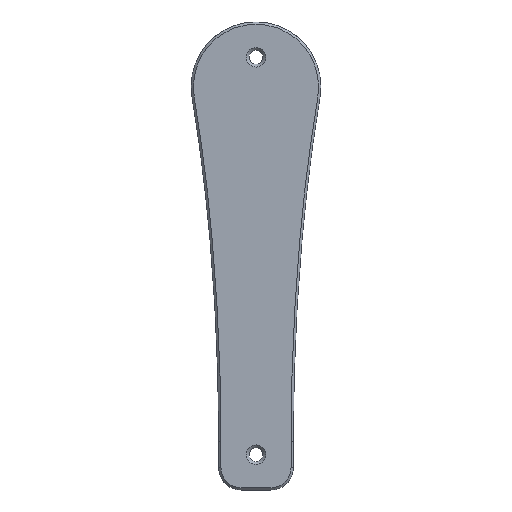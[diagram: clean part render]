
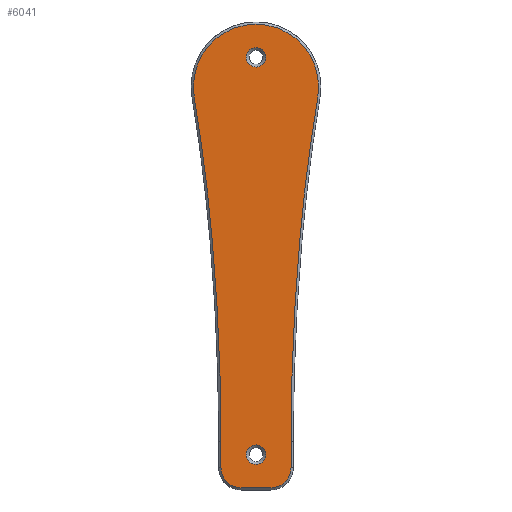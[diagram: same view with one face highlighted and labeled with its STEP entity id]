
A CAD part, front view. The second image highlights one B-rep face of the part: STEP entity #6041.
In plain terms, the highlighted planar face has unit normal (0, -1, 0).
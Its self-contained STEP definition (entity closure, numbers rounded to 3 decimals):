
#19=FACE_BOUND('',#829,.T.);
#20=FACE_BOUND('',#830,.T.);
#27=PLANE('',#6511);
#62=LINE('',#8183,#188);
#66=LINE('',#8195,#192);
#69=LINE('',#8206,#195);
#188=VECTOR('',#6938,10.);
#192=VECTOR('',#6950,10.);
#195=VECTOR('',#6961,10.);
#397=FACE_OUTER_BOUND('',#828,.T.);
#828=EDGE_LOOP('',(#3836,#3837,#3838,#3839,#3840,#3841,#3842,#3843,#3844,
#3845));
#829=EDGE_LOOP('',(#3846));
#830=EDGE_LOOP('',(#3847));
#1817=CIRCLE('',#6482,16.81);
#1820=CIRCLE('',#6486,500.6);
#1821=CIRCLE('',#6488,624.432);
#1824=CIRCLE('',#6493,5.4);
#1825=CIRCLE('',#6496,5.4);
#1828=CIRCLE('',#6501,624.432);
#1829=CIRCLE('',#6503,500.6);
#1832=CIRCLE('',#6512,2.6);
#1833=CIRCLE('',#6513,2.6);
#2138=VERTEX_POINT('',#8159);
#2139=VERTEX_POINT('',#8161);
#2142=VERTEX_POINT('',#8169);
#2144=VERTEX_POINT('',#8174);
#2146=VERTEX_POINT('',#8181);
#2148=VERTEX_POINT('',#8187);
#2150=VERTEX_POINT('',#8193);
#2152=VERTEX_POINT('',#8198);
#2154=VERTEX_POINT('',#8204);
#2156=VERTEX_POINT('',#8211);
#2207=VERTEX_POINT('',#8490);
#2208=VERTEX_POINT('',#8492);
#2718=EDGE_CURVE('',#2138,#2139,#1817,.T.);
#2723=EDGE_CURVE('',#2142,#2138,#1820,.T.);
#2725=EDGE_CURVE('',#2144,#2142,#1821,.T.);
#2729=EDGE_CURVE('',#2146,#2144,#62,.T.);
#2732=EDGE_CURVE('',#2148,#2146,#1824,.T.);
#2735=EDGE_CURVE('',#2150,#2148,#66,.T.);
#2737=EDGE_CURVE('',#2152,#2150,#1825,.T.);
#2740=EDGE_CURVE('',#2154,#2152,#69,.T.);
#2744=EDGE_CURVE('',#2156,#2154,#1828,.T.);
#2745=EDGE_CURVE('',#2139,#2156,#1829,.T.);
#2802=EDGE_CURVE('',#2207,#2207,#1832,.T.);
#2803=EDGE_CURVE('',#2208,#2208,#1833,.T.);
#3836=ORIENTED_EDGE('',*,*,#2718,.F.);
#3837=ORIENTED_EDGE('',*,*,#2723,.F.);
#3838=ORIENTED_EDGE('',*,*,#2725,.F.);
#3839=ORIENTED_EDGE('',*,*,#2729,.F.);
#3840=ORIENTED_EDGE('',*,*,#2732,.F.);
#3841=ORIENTED_EDGE('',*,*,#2735,.F.);
#3842=ORIENTED_EDGE('',*,*,#2737,.F.);
#3843=ORIENTED_EDGE('',*,*,#2740,.F.);
#3844=ORIENTED_EDGE('',*,*,#2744,.F.);
#3845=ORIENTED_EDGE('',*,*,#2745,.F.);
#3846=ORIENTED_EDGE('',*,*,#2802,.F.);
#3847=ORIENTED_EDGE('',*,*,#2803,.F.);
#6041=ADVANCED_FACE('',(#397,#19,#20),#27,.F.);
#6482=AXIS2_PLACEMENT_3D('',#8162,#6915,#6916);
#6486=AXIS2_PLACEMENT_3D('',#8171,#6925,#6926);
#6488=AXIS2_PLACEMENT_3D('',#8176,#6930,#6931);
#6493=AXIS2_PLACEMENT_3D('',#8189,#6944,#6945);
#6496=AXIS2_PLACEMENT_3D('',#8200,#6954,#6955);
#6501=AXIS2_PLACEMENT_3D('',#8213,#6968,#6969);
#6503=AXIS2_PLACEMENT_3D('',#8215,#6972,#6973);
#6511=AXIS2_PLACEMENT_3D('',#8489,#6995,#6996);
#6512=AXIS2_PLACEMENT_3D('',#8491,#6997,#6998);
#6513=AXIS2_PLACEMENT_3D('',#8493,#6999,#7000);
#6915=DIRECTION('center_axis',(0.,1.,0.));
#6916=DIRECTION('ref_axis',(-0.518,0.,0.856));
#6925=DIRECTION('center_axis',(0.,-1.,0.));
#6926=DIRECTION('ref_axis',(0.992,0.,0.125));
#6930=DIRECTION('center_axis',(0.,-1.,0.));
#6931=DIRECTION('ref_axis',(0.99,0.,0.143));
#6938=DIRECTION('',(0.,0.,1.));
#6944=DIRECTION('center_axis',(0.,1.,0.));
#6945=DIRECTION('ref_axis',(-0.707,0.,-0.707));
#6950=DIRECTION('',(-1.,0.,0.));
#6954=DIRECTION('center_axis',(0.,1.,0.));
#6955=DIRECTION('ref_axis',(0.707,0.,-0.707));
#6961=DIRECTION('',(0.,0.,-1.));
#6968=DIRECTION('center_axis',(0.,-1.,0.));
#6969=DIRECTION('ref_axis',(-0.99,0.,0.143));
#6972=DIRECTION('center_axis',(0.,-1.,0.));
#6973=DIRECTION('ref_axis',(-0.992,0.,0.125));
#6995=DIRECTION('center_axis',(0.,1.,0.));
#6996=DIRECTION('ref_axis',(0.,0.,1.));
#6997=DIRECTION('center_axis',(0.,-1.,0.));
#6998=DIRECTION('ref_axis',(1.,0.,0.));
#6999=DIRECTION('center_axis',(0.,-1.,0.));
#7000=DIRECTION('ref_axis',(1.,0.,0.));
#8159=CARTESIAN_POINT('',(7.598,144.038,75.494));
#8161=CARTESIAN_POINT('',(40.768,144.038,75.494));
#8162=CARTESIAN_POINT('Origin',(24.183,144.038,78.237));
#8169=CARTESIAN_POINT('',(12.422,144.038,37.21));
#8171=CARTESIAN_POINT('Origin',(-486.293,144.038,-6.186));
#8174=CARTESIAN_POINT('',(14.773,144.038,-16.92));
#8176=CARTESIAN_POINT('Origin',(-609.659,144.038,-16.92));
#8181=CARTESIAN_POINT('',(14.773,144.038,-24.));
#8183=CARTESIAN_POINT('',(14.773,144.038,48.082));
#8187=CARTESIAN_POINT('',(20.173,144.038,-29.4));
#8189=CARTESIAN_POINT('Origin',(20.173,144.038,-24.));
#8193=CARTESIAN_POINT('',(28.193,144.038,-29.4));
#8195=CARTESIAN_POINT('',(24.183,144.038,-29.4));
#8198=CARTESIAN_POINT('',(33.593,144.038,-24.));
#8200=CARTESIAN_POINT('Origin',(28.193,144.038,-24.));
#8204=CARTESIAN_POINT('',(33.593,144.038,-16.92));
#8206=CARTESIAN_POINT('',(33.593,144.038,48.082));
#8211=CARTESIAN_POINT('',(35.944,144.038,37.21));
#8213=CARTESIAN_POINT('Origin',(658.025,144.038,-16.92));
#8215=CARTESIAN_POINT('Origin',(534.659,144.038,-6.186));
#8489=CARTESIAN_POINT('Origin',(24.183,144.038,32.823));
#8490=CARTESIAN_POINT('',(21.583,144.038,-20.514));
#8491=CARTESIAN_POINT('Origin',(24.183,144.038,-20.514));
#8492=CARTESIAN_POINT('',(21.583,144.038,86.161));
#8493=CARTESIAN_POINT('Origin',(24.183,144.038,86.161));
